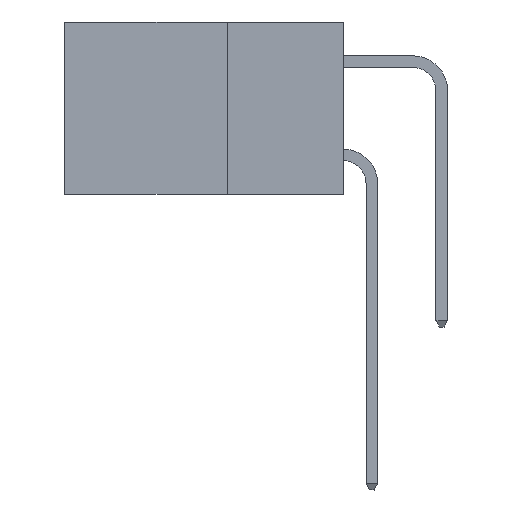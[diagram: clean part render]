
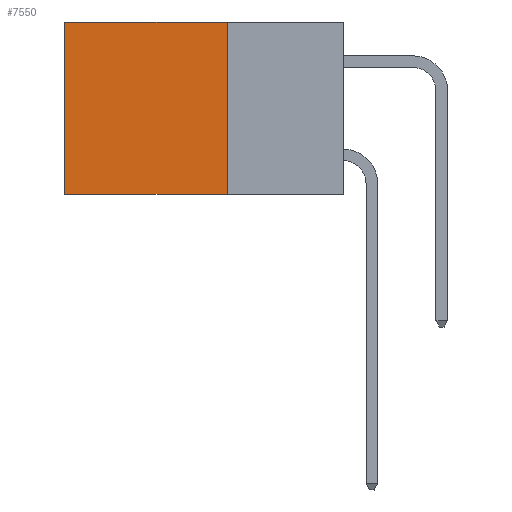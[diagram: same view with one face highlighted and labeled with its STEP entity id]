
A CAD part, left-side view. The second image highlights one B-rep face of the part: STEP entity #7550.
In plain terms, the highlighted planar face has unit normal (-1, 0, 0).
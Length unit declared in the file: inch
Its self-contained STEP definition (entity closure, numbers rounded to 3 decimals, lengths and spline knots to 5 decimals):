
#755 = EDGE_CURVE ( 'NONE', #4655, #9970, #1137, .T. ) ;
#786 = LINE ( 'NONE', #2072, #6805 ) ;
#1137 = LINE ( 'NONE', #5808, #8336 ) ;
#1407 = LINE ( 'NONE', #9056, #4964 ) ;
#1734 = ORIENTED_EDGE ( 'NONE', *, *, #2614, .F. ) ;
#2023 = ORIENTED_EDGE ( 'NONE', *, *, #755, .F. ) ;
#2072 = CARTESIAN_POINT ( 'NONE',  ( 0.298, 0.25, 0. ) ) ;
#2397 = CARTESIAN_POINT ( 'NONE',  ( 0.298, 0.6, 0. ) ) ;
#2614 = EDGE_CURVE ( 'NONE', #3105, #4655, #1407, .T. ) ;
#2634 = CARTESIAN_POINT ( 'NONE',  ( 0.298, 0.25, -0.37 ) ) ;
#3001 = EDGE_CURVE ( 'NONE', #3105, #6754, #786, .T. ) ;
#3105 = VERTEX_POINT ( 'NONE', #9912 ) ;
#4205 = DIRECTION ( 'NONE',  ( 1., 0., 0. ) ) ;
#4655 = VERTEX_POINT ( 'NONE', #2634 ) ;
#4964 = VECTOR ( 'NONE', #6845, 39.37008 ) ;
#5808 = CARTESIAN_POINT ( 'NONE',  ( 0.298, 0.25, -0.37 ) ) ;
#6107 = DIRECTION ( 'NONE',  ( 0., 0., -1. ) ) ;
#6200 = LINE ( 'NONE', #2397, #10089 ) ;
#6418 = ORIENTED_EDGE ( 'NONE', *, *, #9466, .T. ) ;
#6754 = VERTEX_POINT ( 'NONE', #9164 ) ;
#6805 = VECTOR ( 'NONE', #10624, 39.37008 ) ;
#6845 = DIRECTION ( 'NONE',  ( 0., 0., -1. ) ) ;
#7261 = AXIS2_PLACEMENT_3D ( 'NONE', #8010, #4205, #6107 ) ;
#7507 = CARTESIAN_POINT ( 'NONE',  ( 0.298, 0.6, -0.37 ) ) ;
#7550 = ADVANCED_FACE ( 'NONE', ( #10927 ), #11874, .F. ) ;
#7838 = EDGE_LOOP ( 'NONE', ( #6418, #2023, #1734, #11375 ) ) ;
#8010 = CARTESIAN_POINT ( 'NONE',  ( 0.298, 0.25, 0. ) ) ;
#8203 = DIRECTION ( 'NONE',  ( 0., 0., -1. ) ) ;
#8336 = VECTOR ( 'NONE', #10673, 39.37008 ) ;
#9056 = CARTESIAN_POINT ( 'NONE',  ( 0.298, 0.25, 0. ) ) ;
#9164 = CARTESIAN_POINT ( 'NONE',  ( 0.298, 0.6, 0. ) ) ;
#9466 = EDGE_CURVE ( 'NONE', #6754, #9970, #6200, .T. ) ;
#9912 = CARTESIAN_POINT ( 'NONE',  ( 0.298, 0.25, 0. ) ) ;
#9970 = VERTEX_POINT ( 'NONE', #7507 ) ;
#10089 = VECTOR ( 'NONE', #8203, 39.37008 ) ;
#10624 = DIRECTION ( 'NONE',  ( 0., 1., 0. ) ) ;
#10673 = DIRECTION ( 'NONE',  ( 0., 1., 0. ) ) ;
#10927 = FACE_OUTER_BOUND ( 'NONE', #7838, .T. ) ;
#11375 = ORIENTED_EDGE ( 'NONE', *, *, #3001, .T. ) ;
#11874 = PLANE ( 'NONE',  #7261 ) ;
